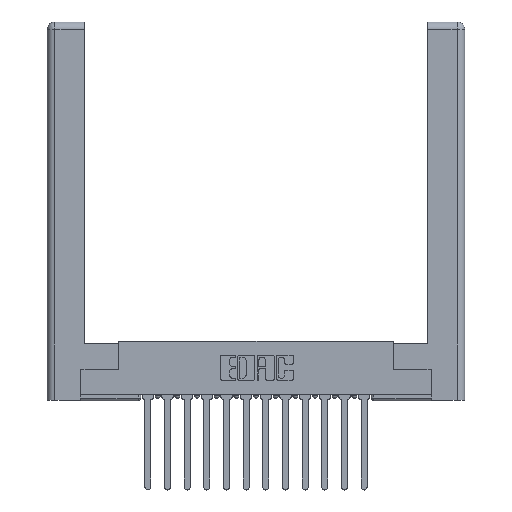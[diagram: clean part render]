
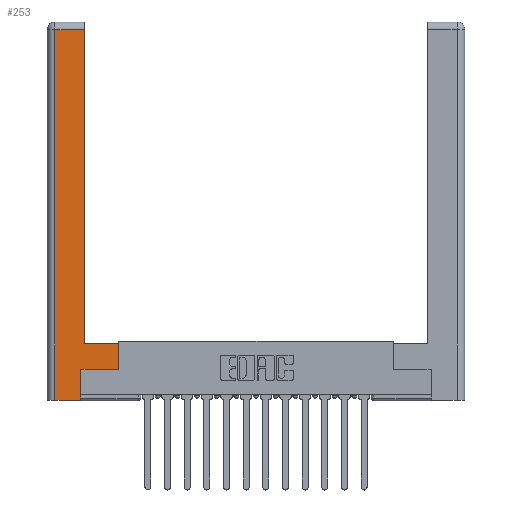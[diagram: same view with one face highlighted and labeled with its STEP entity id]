
A CAD part, top view. The second image highlights one B-rep face of the part: STEP entity #253.
In plain terms, the highlighted planar face has unit normal (0, 0, 1).
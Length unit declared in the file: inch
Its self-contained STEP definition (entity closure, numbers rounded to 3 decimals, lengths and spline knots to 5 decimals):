
#117 = CARTESIAN_POINT ( 'NONE',  ( 0.295, 2.94, 0. ) ) ;
#253 = ADVANCED_FACE ( 'NONE', ( #6290 ), #5073, .F. ) ;
#291 = CARTESIAN_POINT ( 'NONE',  ( 0.265, 0.245, 0. ) ) ;
#504 = CARTESIAN_POINT ( 'NONE',  ( 0.265, 0.245, 0. ) ) ;
#660 = CARTESIAN_POINT ( 'NONE',  ( 0.295, 0.45, 0. ) ) ;
#739 = EDGE_CURVE ( 'NONE', #7870, #3518, #5072, .T. ) ;
#777 = LINE ( 'NONE', #5958, #16383 ) ;
#1612 = VERTEX_POINT ( 'NONE', #117 ) ;
#1848 = EDGE_CURVE ( 'NONE', #14485, #11294, #3363, .T. ) ;
#2715 = VERTEX_POINT ( 'NONE', #4266 ) ;
#2919 = CARTESIAN_POINT ( 'NONE',  ( 0.565, 0.45, 0. ) ) ;
#3102 = ORIENTED_EDGE ( 'NONE', *, *, #14512, .T. ) ;
#3187 = DIRECTION ( 'NONE',  ( 1., 0., 0. ) ) ;
#3363 = LINE ( 'NONE', #7160, #3979 ) ;
#3385 = CARTESIAN_POINT ( 'NONE',  ( 0.295, 0.45, 0. ) ) ;
#3518 = VERTEX_POINT ( 'NONE', #660 ) ;
#3749 = LINE ( 'NONE', #2919, #15696 ) ;
#3979 = VECTOR ( 'NONE', #11260, 39.37008 ) ;
#4266 = CARTESIAN_POINT ( 'NONE',  ( 0.265, 0., 0. ) ) ;
#4896 = EDGE_LOOP ( 'NONE', ( #5805, #14469, #6795, #3102, #8329, #9420, #16838, #8165 ) ) ;
#5072 = LINE ( 'NONE', #3385, #11671 ) ;
#5073 = PLANE ( 'NONE',  #15436 ) ;
#5110 = CARTESIAN_POINT ( 'NONE',  ( 0.265, 0., 0. ) ) ;
#5805 = ORIENTED_EDGE ( 'NONE', *, *, #12512, .T. ) ;
#5958 = CARTESIAN_POINT ( 'NONE',  ( 0.565, 0.245, 0. ) ) ;
#6180 = VECTOR ( 'NONE', #11074, 39.37008 ) ;
#6290 = FACE_OUTER_BOUND ( 'NONE', #4896, .T. ) ;
#6359 = VERTEX_POINT ( 'NONE', #504 ) ;
#6527 = CARTESIAN_POINT ( 'NONE',  ( 0.0615, 2.94, 0. ) ) ;
#6593 = LINE ( 'NONE', #16267, #6180 ) ;
#6795 = ORIENTED_EDGE ( 'NONE', *, *, #1848, .T. ) ;
#7160 = CARTESIAN_POINT ( 'NONE',  ( 0.0615, 0., 0. ) ) ;
#7609 = CARTESIAN_POINT ( 'NONE',  ( 0., 0., 0. ) ) ;
#7870 = VERTEX_POINT ( 'NONE', #10028 ) ;
#8165 = ORIENTED_EDGE ( 'NONE', *, *, #739, .T. ) ;
#8329 = ORIENTED_EDGE ( 'NONE', *, *, #16966, .T. ) ;
#8406 = EDGE_CURVE ( 'NONE', #6359, #11023, #777, .T. ) ;
#8652 = DIRECTION ( 'NONE',  ( -1., 0., 0. ) ) ;
#9420 = ORIENTED_EDGE ( 'NONE', *, *, #8406, .T. ) ;
#9574 = DIRECTION ( 'NONE',  ( 0., 0., -1. ) ) ;
#9624 = DIRECTION ( 'NONE',  ( -1., 0., 0. ) ) ;
#9794 = DIRECTION ( 'NONE',  ( 0., 1., 0. ) ) ;
#9807 = VECTOR ( 'NONE', #9794, 39.37008 ) ;
#9923 = EDGE_CURVE ( 'NONE', #1612, #14485, #6593, .T. ) ;
#10028 = CARTESIAN_POINT ( 'NONE',  ( 0.565, 0.45, 0. ) ) ;
#10787 = LINE ( 'NONE', #291, #13641 ) ;
#11023 = VERTEX_POINT ( 'NONE', #16498 ) ;
#11074 = DIRECTION ( 'NONE',  ( -1., 0., 0. ) ) ;
#11260 = DIRECTION ( 'NONE',  ( 0., -1., 0. ) ) ;
#11294 = VERTEX_POINT ( 'NONE', #16111 ) ;
#11671 = VECTOR ( 'NONE', #8652, 39.37008 ) ;
#12120 = DIRECTION ( 'NONE',  ( 0., 1., 0. ) ) ;
#12438 = LINE ( 'NONE', #14921, #9807 ) ;
#12512 = EDGE_CURVE ( 'NONE', #3518, #1612, #12438, .T. ) ;
#13013 = VECTOR ( 'NONE', #15676, 39.37008 ) ;
#13330 = DIRECTION ( 'NONE',  ( 0., 1., 0. ) ) ;
#13641 = VECTOR ( 'NONE', #13330, 39.37008 ) ;
#13993 = EDGE_CURVE ( 'NONE', #11023, #7870, #3749, .T. ) ;
#14469 = ORIENTED_EDGE ( 'NONE', *, *, #9923, .T. ) ;
#14485 = VERTEX_POINT ( 'NONE', #6527 ) ;
#14512 = EDGE_CURVE ( 'NONE', #11294, #2715, #16475, .T. ) ;
#14921 = CARTESIAN_POINT ( 'NONE',  ( 0.295, 3., 0. ) ) ;
#15436 = AXIS2_PLACEMENT_3D ( 'NONE', #7609, #9574, #9624 ) ;
#15676 = DIRECTION ( 'NONE',  ( 1., 0., 0. ) ) ;
#15696 = VECTOR ( 'NONE', #12120, 39.37008 ) ;
#16111 = CARTESIAN_POINT ( 'NONE',  ( 0.0615, 0., 0. ) ) ;
#16267 = CARTESIAN_POINT ( 'NONE',  ( 0.0615, 2.94, 0. ) ) ;
#16383 = VECTOR ( 'NONE', #3187, 39.37008 ) ;
#16475 = LINE ( 'NONE', #5110, #13013 ) ;
#16498 = CARTESIAN_POINT ( 'NONE',  ( 0.565, 0.245, 0. ) ) ;
#16838 = ORIENTED_EDGE ( 'NONE', *, *, #13993, .T. ) ;
#16966 = EDGE_CURVE ( 'NONE', #2715, #6359, #10787, .T. ) ;
